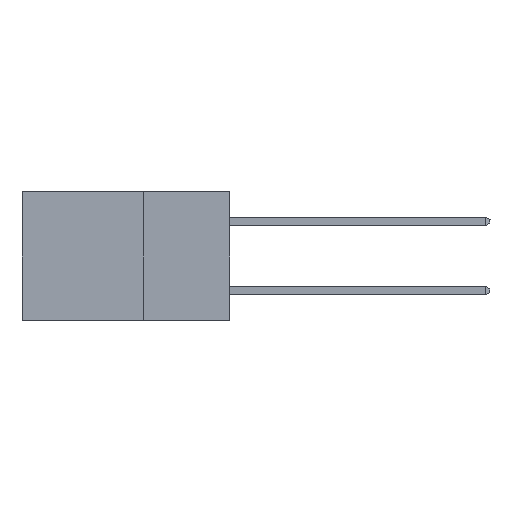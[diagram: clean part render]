
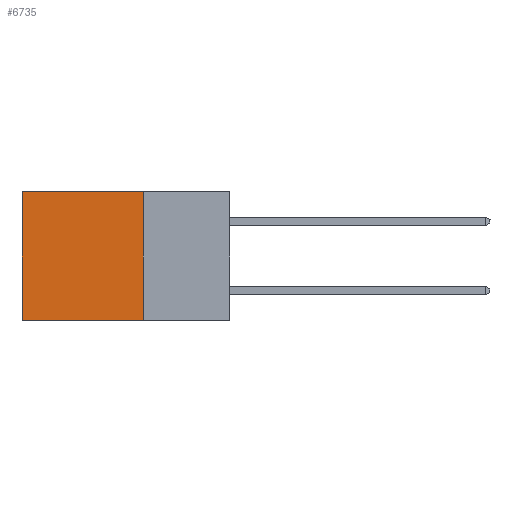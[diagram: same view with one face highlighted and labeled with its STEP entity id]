
A CAD part, left-side view. The second image highlights one B-rep face of the part: STEP entity #6735.
In plain terms, the highlighted planar face has unit normal (-1, 0, 0).
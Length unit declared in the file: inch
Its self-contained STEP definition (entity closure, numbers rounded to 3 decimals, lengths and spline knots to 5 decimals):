
#808 = VECTOR ( 'NONE', #4467, 39.37008 ) ;
#1356 = CARTESIAN_POINT ( 'NONE',  ( 0.2615, 0.6, -0.37 ) ) ;
#1830 = CARTESIAN_POINT ( 'NONE',  ( 0.2615, 0.25, -0.37 ) ) ;
#1881 = DIRECTION ( 'NONE',  ( 0., 1., 0. ) ) ;
#1894 = DIRECTION ( 'NONE',  ( 0., 0., -1. ) ) ;
#1995 = ORIENTED_EDGE ( 'NONE', *, *, #10956, .F. ) ;
#2182 = ORIENTED_EDGE ( 'NONE', *, *, #10667, .T. ) ;
#2398 = DIRECTION ( 'NONE',  ( 0., 0., -1. ) ) ;
#3007 = ORIENTED_EDGE ( 'NONE', *, *, #3799, .T. ) ;
#3464 = VERTEX_POINT ( 'NONE', #8280 ) ;
#3799 = EDGE_CURVE ( 'NONE', #9872, #5452, #4609, .T. ) ;
#4098 = LINE ( 'NONE', #9320, #5241 ) ;
#4112 = VECTOR ( 'NONE', #1881, 39.37008 ) ;
#4467 = DIRECTION ( 'NONE',  ( 0., 1., 0. ) ) ;
#4609 = LINE ( 'NONE', #1356, #5973 ) ;
#4869 = EDGE_LOOP ( 'NONE', ( #3007, #4954, #1995, #2182 ) ) ;
#4954 = ORIENTED_EDGE ( 'NONE', *, *, #9705, .F. ) ;
#5241 = VECTOR ( 'NONE', #9239, 39.37008 ) ;
#5452 = VERTEX_POINT ( 'NONE', #12772 ) ;
#5578 = LINE ( 'NONE', #11955, #808 ) ;
#5973 = VECTOR ( 'NONE', #2398, 39.37008 ) ;
#5974 = CARTESIAN_POINT ( 'NONE',  ( 0.2615, 0.25, -0.37 ) ) ;
#6300 = CARTESIAN_POINT ( 'NONE',  ( 0.2615, 0.6, 0. ) ) ;
#6735 = ADVANCED_FACE ( 'NONE', ( #11337 ), #10452, .F. ) ;
#7268 = AXIS2_PLACEMENT_3D ( 'NONE', #1830, #9334, #1894 ) ;
#8055 = CARTESIAN_POINT ( 'NONE',  ( 0.2615, 0.25, -0.37 ) ) ;
#8280 = CARTESIAN_POINT ( 'NONE',  ( 0.2615, 0.25, 0. ) ) ;
#9239 = DIRECTION ( 'NONE',  ( 0., 0., -1. ) ) ;
#9320 = CARTESIAN_POINT ( 'NONE',  ( 0.2615, 0.25, -0.37 ) ) ;
#9334 = DIRECTION ( 'NONE',  ( 1., 0., 0. ) ) ;
#9600 = VERTEX_POINT ( 'NONE', #8055 ) ;
#9705 = EDGE_CURVE ( 'NONE', #9600, #5452, #11248, .T. ) ;
#9872 = VERTEX_POINT ( 'NONE', #6300 ) ;
#10452 = PLANE ( 'NONE',  #7268 ) ;
#10667 = EDGE_CURVE ( 'NONE', #3464, #9872, #5578, .T. ) ;
#10956 = EDGE_CURVE ( 'NONE', #3464, #9600, #4098, .T. ) ;
#11248 = LINE ( 'NONE', #5974, #4112 ) ;
#11337 = FACE_OUTER_BOUND ( 'NONE', #4869, .T. ) ;
#11955 = CARTESIAN_POINT ( 'NONE',  ( 0.2615, 0.25, 0. ) ) ;
#12772 = CARTESIAN_POINT ( 'NONE',  ( 0.2615, 0.6, -0.37 ) ) ;
